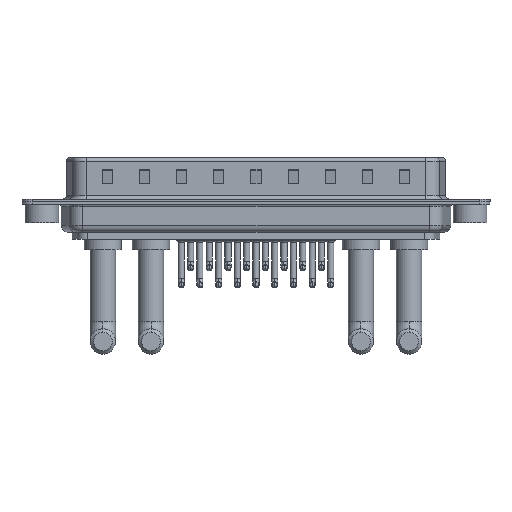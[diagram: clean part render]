
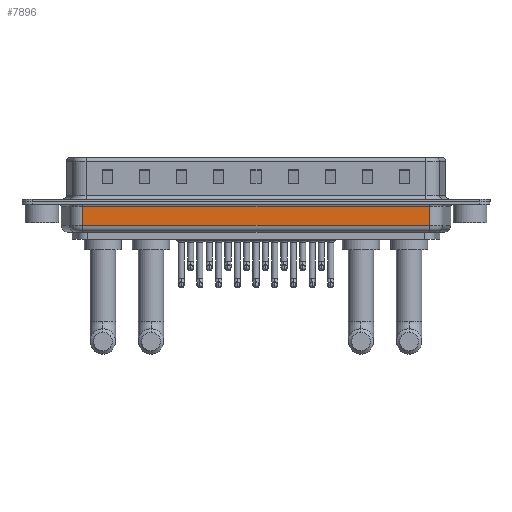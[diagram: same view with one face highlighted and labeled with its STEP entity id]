
A CAD part, front view. The second image highlights one B-rep face of the part: STEP entity #7896.
In plain terms, the highlighted planar face has unit normal (0, -1, 0).
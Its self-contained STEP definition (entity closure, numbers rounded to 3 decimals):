
#430 = EDGE_CURVE ( 'NONE', #22666, #24799, #6763, .T. ) ;
#518 = FACE_OUTER_BOUND ( 'NONE', #19727, .T. ) ;
#1038 = VECTOR ( 'NONE', #19319, 1000. ) ;
#1791 = ORIENTED_EDGE ( 'NONE', *, *, #430, .F. ) ;
#2667 = CARTESIAN_POINT ( 'NONE',  ( 6.031, -5.35, -4.5 ) ) ;
#4816 = LINE ( 'NONE', #8627, #22137 ) ;
#5009 = EDGE_CURVE ( 'NONE', #5276, #24605, #4816, .T. ) ;
#5276 = VERTEX_POINT ( 'NONE', #18634 ) ;
#6763 = LINE ( 'NONE', #2667, #13847 ) ;
#6766 = DIRECTION ( 'NONE',  ( 0., 1., 0. ) ) ;
#7145 = DIRECTION ( 'NONE',  ( -1., 0., 0. ) ) ;
#7896 = ADVANCED_FACE ( 'NONE', ( #518 ), #8792, .F. ) ;
#8583 = EDGE_CURVE ( 'NONE', #22666, #5276, #19449, .T. ) ;
#8627 = CARTESIAN_POINT ( 'NONE',  ( 57.469, -5.35, -4.5 ) ) ;
#8792 = PLANE ( 'NONE',  #25363 ) ;
#10760 = DIRECTION ( 'NONE',  ( -1., 0., 0. ) ) ;
#10790 = DIRECTION ( 'NONE',  ( 0., 0., 1. ) ) ;
#11082 = DIRECTION ( 'NONE',  ( 0., 0., 1. ) ) ;
#12238 = ORIENTED_EDGE ( 'NONE', *, *, #24931, .T. ) ;
#12765 = CARTESIAN_POINT ( 'NONE',  ( 6.031, -5.35, -0.65 ) ) ;
#13847 = VECTOR ( 'NONE', #11082, 1000. ) ;
#14809 = LINE ( 'NONE', #12765, #17514 ) ;
#15227 = CARTESIAN_POINT ( 'NONE',  ( 57.469, -5.35, -0.65 ) ) ;
#15678 = ORIENTED_EDGE ( 'NONE', *, *, #8583, .T. ) ;
#17047 = CARTESIAN_POINT ( 'NONE',  ( 6.031, -5.35, -4.5 ) ) ;
#17514 = VECTOR ( 'NONE', #10760, 1000. ) ;
#18634 = CARTESIAN_POINT ( 'NONE',  ( 57.469, -5.35, -3.5 ) ) ;
#19050 = CARTESIAN_POINT ( 'NONE',  ( 6.031, -5.35, -3.5 ) ) ;
#19319 = DIRECTION ( 'NONE',  ( 1., 0., 0. ) ) ;
#19449 = LINE ( 'NONE', #19050, #1038 ) ;
#19548 = ORIENTED_EDGE ( 'NONE', *, *, #5009, .T. ) ;
#19727 = EDGE_LOOP ( 'NONE', ( #1791, #15678, #19548, #12238 ) ) ;
#22137 = VECTOR ( 'NONE', #10790, 1000. ) ;
#22387 = CARTESIAN_POINT ( 'NONE',  ( 6.031, -5.35, -3.5 ) ) ;
#22666 = VERTEX_POINT ( 'NONE', #22387 ) ;
#24605 = VERTEX_POINT ( 'NONE', #15227 ) ;
#24799 = VERTEX_POINT ( 'NONE', #26646 ) ;
#24931 = EDGE_CURVE ( 'NONE', #24605, #24799, #14809, .T. ) ;
#25363 = AXIS2_PLACEMENT_3D ( 'NONE', #17047, #6766, #7145 ) ;
#26646 = CARTESIAN_POINT ( 'NONE',  ( 6.031, -5.35, -0.65 ) ) ;
